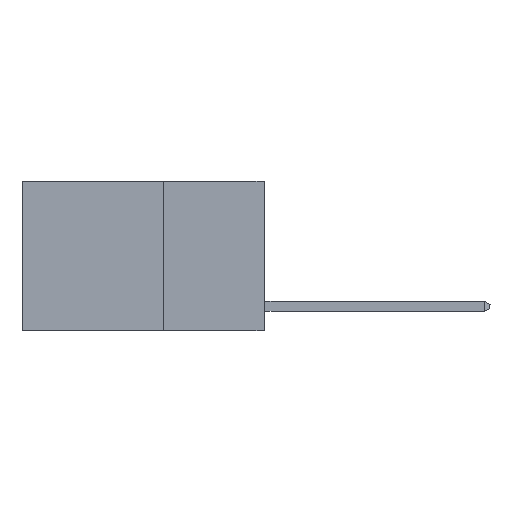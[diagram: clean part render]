
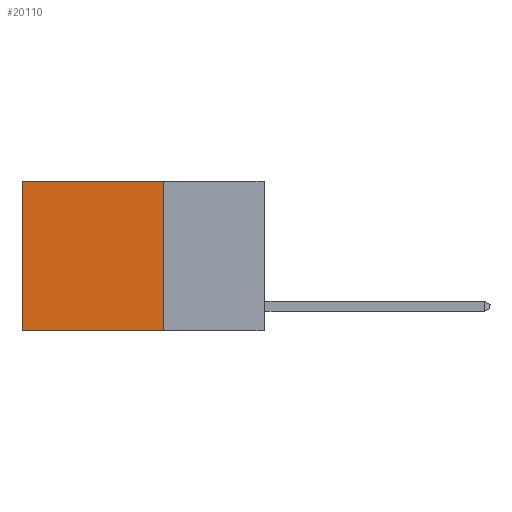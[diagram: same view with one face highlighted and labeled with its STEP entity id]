
A CAD part, left-side view. The second image highlights one B-rep face of the part: STEP entity #20110.
In plain terms, the highlighted planar face has unit normal (-1, 0, 0).
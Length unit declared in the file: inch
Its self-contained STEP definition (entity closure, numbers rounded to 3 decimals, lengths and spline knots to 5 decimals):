
#38 = CARTESIAN_POINT ( 'NONE',  ( 0.2625, 0.6, 0. ) ) ;
#373 = EDGE_CURVE ( 'NONE', #5520, #9865, #10898, .T. ) ;
#416 = EDGE_LOOP ( 'NONE', ( #14901, #6421, #9356, #17621 ) ) ;
#536 = CARTESIAN_POINT ( 'NONE',  ( 0.2625, 0.25, 0. ) ) ;
#1401 = CARTESIAN_POINT ( 'NONE',  ( 0.2625, 0.25, -0.37 ) ) ;
#2502 = DIRECTION ( 'NONE',  ( 0., 1., 0. ) ) ;
#3182 = DIRECTION ( 'NONE',  ( 0., 0., -1. ) ) ;
#3517 = EDGE_CURVE ( 'NONE', #16244, #3580, #16086, .T. ) ;
#3534 = DIRECTION ( 'NONE',  ( 0., 1., 0. ) ) ;
#3580 = VERTEX_POINT ( 'NONE', #19744 ) ;
#5520 = VERTEX_POINT ( 'NONE', #536 ) ;
#5931 = EDGE_CURVE ( 'NONE', #5520, #16244, #12318, .T. ) ;
#6184 = VECTOR ( 'NONE', #2502, 39.37008 ) ;
#6421 = ORIENTED_EDGE ( 'NONE', *, *, #22440, .F. ) ;
#9303 = CARTESIAN_POINT ( 'NONE',  ( 0.2625, 0.25, 0. ) ) ;
#9356 = ORIENTED_EDGE ( 'NONE', *, *, #373, .F. ) ;
#9865 = VERTEX_POINT ( 'NONE', #1401 ) ;
#10898 = LINE ( 'NONE', #14815, #21273 ) ;
#11224 = FACE_OUTER_BOUND ( 'NONE', #416, .T. ) ;
#11372 = CARTESIAN_POINT ( 'NONE',  ( 0.2625, 0.25, -0.37 ) ) ;
#12318 = LINE ( 'NONE', #9303, #15497 ) ;
#13161 = LINE ( 'NONE', #11372, #6184 ) ;
#14815 = CARTESIAN_POINT ( 'NONE',  ( 0.2625, 0.25, 0. ) ) ;
#14901 = ORIENTED_EDGE ( 'NONE', *, *, #3517, .T. ) ;
#15497 = VECTOR ( 'NONE', #3534, 39.37008 ) ;
#15971 = DIRECTION ( 'NONE',  ( 0., 0., -1. ) ) ;
#16086 = LINE ( 'NONE', #38, #22556 ) ;
#16244 = VERTEX_POINT ( 'NONE', #16313 ) ;
#16313 = CARTESIAN_POINT ( 'NONE',  ( 0.2625, 0.6, 0. ) ) ;
#17621 = ORIENTED_EDGE ( 'NONE', *, *, #5931, .T. ) ;
#18251 = DIRECTION ( 'NONE',  ( 0., 0., -1. ) ) ;
#18461 = PLANE ( 'NONE',  #19452 ) ;
#19395 = DIRECTION ( 'NONE',  ( 1., 0., 0. ) ) ;
#19452 = AXIS2_PLACEMENT_3D ( 'NONE', #19510, #19395, #3182 ) ;
#19510 = CARTESIAN_POINT ( 'NONE',  ( 0.2625, 0.25, 0. ) ) ;
#19744 = CARTESIAN_POINT ( 'NONE',  ( 0.2625, 0.6, -0.37 ) ) ;
#20110 = ADVANCED_FACE ( 'NONE', ( #11224 ), #18461, .F. ) ;
#21273 = VECTOR ( 'NONE', #18251, 39.37008 ) ;
#22440 = EDGE_CURVE ( 'NONE', #9865, #3580, #13161, .T. ) ;
#22556 = VECTOR ( 'NONE', #15971, 39.37008 ) ;
